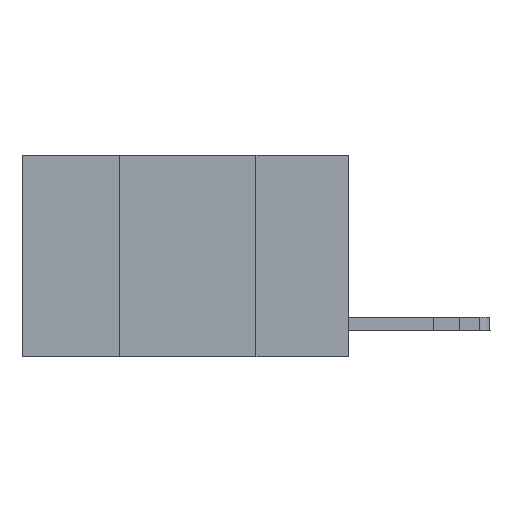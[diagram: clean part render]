
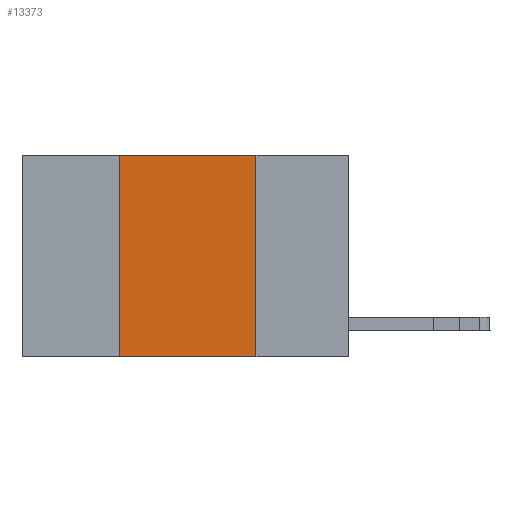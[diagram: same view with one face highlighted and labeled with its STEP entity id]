
A CAD part, left-side view. The second image highlights one B-rep face of the part: STEP entity #13373.
In plain terms, the highlighted planar face has unit normal (-1, 0, 0).
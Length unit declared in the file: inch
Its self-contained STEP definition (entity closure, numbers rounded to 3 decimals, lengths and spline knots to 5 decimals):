
#899 = DIRECTION ( 'NONE',  ( 0., -1., 0. ) ) ;
#969 = DIRECTION ( 'NONE',  ( 0., 0., -1. ) ) ;
#1497 = CARTESIAN_POINT ( 'NONE',  ( 0., 0.42, 0. ) ) ;
#1692 = VERTEX_POINT ( 'NONE', #1497 ) ;
#1716 = DIRECTION ( 'NONE',  ( 0., 0., 1. ) ) ;
#1721 = CARTESIAN_POINT ( 'NONE',  ( 0., 0.17, -0.37 ) ) ;
#1856 = VERTEX_POINT ( 'NONE', #1721 ) ;
#2722 = EDGE_CURVE ( 'NONE', #6747, #1692, #14601, .T. ) ;
#3295 = CARTESIAN_POINT ( 'NONE',  ( 0., 0.6, -0.37 ) ) ;
#4588 = LINE ( 'NONE', #17371, #9882 ) ;
#4613 = EDGE_CURVE ( 'NONE', #5355, #1856, #4588, .T. ) ;
#5081 = LINE ( 'NONE', #3295, #8818 ) ;
#5096 = CARTESIAN_POINT ( 'NONE',  ( 0., 0.42, 0. ) ) ;
#5355 = VERTEX_POINT ( 'NONE', #14441 ) ;
#6303 = LINE ( 'NONE', #19152, #7146 ) ;
#6747 = VERTEX_POINT ( 'NONE', #18451 ) ;
#7146 = VECTOR ( 'NONE', #899, 39.37008 ) ;
#8818 = VECTOR ( 'NONE', #17898, 39.37008 ) ;
#9237 = EDGE_CURVE ( 'NONE', #6747, #1856, #5081, .T. ) ;
#9882 = VECTOR ( 'NONE', #969, 39.37008 ) ;
#9903 = ORIENTED_EDGE ( 'NONE', *, *, #9237, .T. ) ;
#11179 = PLANE ( 'NONE',  #12620 ) ;
#12620 = AXIS2_PLACEMENT_3D ( 'NONE', #16361, #20619, #18583 ) ;
#13373 = ADVANCED_FACE ( 'NONE', ( #16844 ), #11179, .F. ) ;
#14441 = CARTESIAN_POINT ( 'NONE',  ( 0., 0.17, 0. ) ) ;
#14601 = LINE ( 'NONE', #5096, #20508 ) ;
#16361 = CARTESIAN_POINT ( 'NONE',  ( 0., 0.6, 0. ) ) ;
#16844 = FACE_OUTER_BOUND ( 'NONE', #20269, .T. ) ;
#17371 = CARTESIAN_POINT ( 'NONE',  ( 0., 0.17, 0. ) ) ;
#17898 = DIRECTION ( 'NONE',  ( 0., -1., 0. ) ) ;
#18451 = CARTESIAN_POINT ( 'NONE',  ( 0., 0.42, -0.37 ) ) ;
#18485 = ORIENTED_EDGE ( 'NONE', *, *, #4613, .F. ) ;
#18583 = DIRECTION ( 'NONE',  ( 0., 0., -1. ) ) ;
#19152 = CARTESIAN_POINT ( 'NONE',  ( 0., 0.6, 0. ) ) ;
#19172 = ORIENTED_EDGE ( 'NONE', *, *, #21906, .F. ) ;
#20269 = EDGE_LOOP ( 'NONE', ( #18485, #19172, #20664, #9903 ) ) ;
#20508 = VECTOR ( 'NONE', #1716, 39.37008 ) ;
#20619 = DIRECTION ( 'NONE',  ( 1., 0., 0. ) ) ;
#20664 = ORIENTED_EDGE ( 'NONE', *, *, #2722, .F. ) ;
#21906 = EDGE_CURVE ( 'NONE', #1692, #5355, #6303, .T. ) ;
